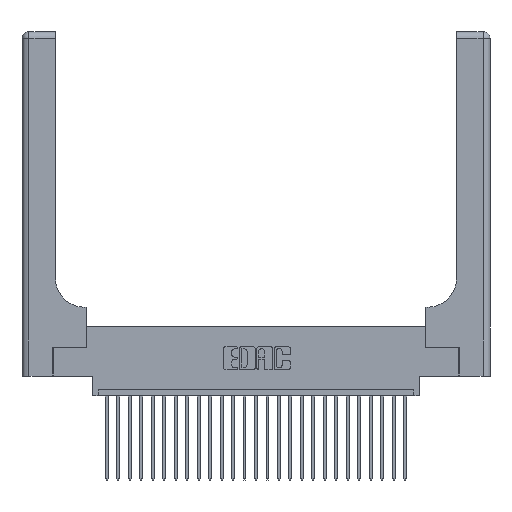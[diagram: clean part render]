
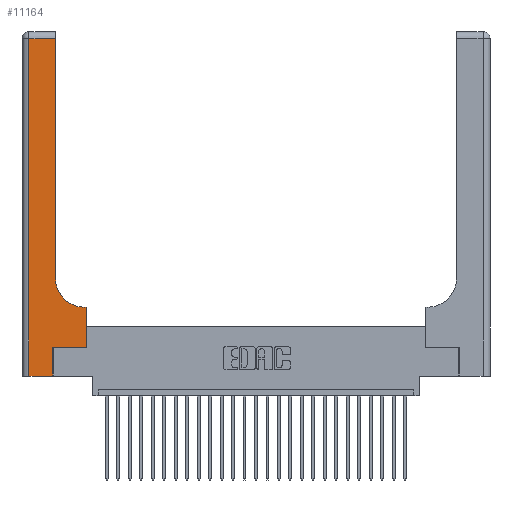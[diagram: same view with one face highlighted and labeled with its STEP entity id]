
A CAD part, top view. The second image highlights one B-rep face of the part: STEP entity #11164.
In plain terms, the highlighted planar face has unit normal (0, 0, 1).
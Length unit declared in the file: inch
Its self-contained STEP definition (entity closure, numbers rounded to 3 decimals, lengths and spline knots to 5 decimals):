
#242 = ORIENTED_EDGE ( 'NONE', *, *, #26718, .T. ) ;
#314 = ORIENTED_EDGE ( 'NONE', *, *, #1433, .T. ) ;
#430 = FACE_OUTER_BOUND ( 'NONE', #13887, .T. ) ;
#598 = EDGE_CURVE ( 'NONE', #5281, #12562, #3356, .T. ) ;
#743 = CIRCLE ( 'NONE', #6125, 0.25 ) ;
#753 = CARTESIAN_POINT ( 'NONE',  ( 0.269, 0., 0.37 ) ) ;
#837 = DIRECTION ( 'NONE',  ( 0., 1., 0. ) ) ;
#1378 = DIRECTION ( 'NONE',  ( -1., 0., 0. ) ) ;
#1433 = EDGE_CURVE ( 'NONE', #15170, #6811, #19307, .T. ) ;
#3356 = LINE ( 'NONE', #22307, #25437 ) ;
#3408 = LINE ( 'NONE', #11684, #14414 ) ;
#4269 = EDGE_CURVE ( 'NONE', #12562, #13322, #24216, .T. ) ;
#4612 = CARTESIAN_POINT ( 'NONE',  ( 0.269, 0.25, 0.37 ) ) ;
#4697 = AXIS2_PLACEMENT_3D ( 'NONE', #5460, #16264, #18452 ) ;
#4701 = ORIENTED_EDGE ( 'NONE', *, *, #17840, .T. ) ;
#5043 = ORIENTED_EDGE ( 'NONE', *, *, #20445, .T. ) ;
#5281 = VERTEX_POINT ( 'NONE', #20880 ) ;
#5336 = CARTESIAN_POINT ( 'NONE',  ( 0.2915, 0.85, 0.37 ) ) ;
#5461 = VERTEX_POINT ( 'NONE', #25775 ) ;
#5460 = CARTESIAN_POINT ( 'NONE',  ( 0., 3., 0.37 ) ) ;
#5599 = CARTESIAN_POINT ( 'NONE',  ( 0., 0., 0.37 ) ) ;
#6125 = AXIS2_PLACEMENT_3D ( 'NONE', #19840, #26331, #11038 ) ;
#6410 = LINE ( 'NONE', #22202, #8734 ) ;
#6789 = VECTOR ( 'NONE', #22715, 39.37008 ) ;
#6811 = VERTEX_POINT ( 'NONE', #27147 ) ;
#8466 = ORIENTED_EDGE ( 'NONE', *, *, #4269, .T. ) ;
#8581 = CARTESIAN_POINT ( 'NONE',  ( 0.06, 0., 0.37 ) ) ;
#8734 = VECTOR ( 'NONE', #837, 39.37008 ) ;
#10805 = CARTESIAN_POINT ( 'NONE',  ( 0.5585, 0.6, 0.37 ) ) ;
#11038 = DIRECTION ( 'NONE',  ( 1., 0., 0. ) ) ;
#11164 = ADVANCED_FACE ( 'NONE', ( #430 ), #22750, .F. ) ;
#11684 = CARTESIAN_POINT ( 'NONE',  ( 0., 2.94, 0.37 ) ) ;
#12562 = VERTEX_POINT ( 'NONE', #8581 ) ;
#12985 = CARTESIAN_POINT ( 'NONE',  ( 0.2915, 0.6, 0.37 ) ) ;
#13123 = VECTOR ( 'NONE', #14630, 39.37008 ) ;
#13152 = ORIENTED_EDGE ( 'NONE', *, *, #15924, .T. ) ;
#13322 = VERTEX_POINT ( 'NONE', #753 ) ;
#13780 = VECTOR ( 'NONE', #22208, 39.37008 ) ;
#13887 = EDGE_LOOP ( 'NONE', ( #14535, #24738, #14708, #8466, #242, #314, #13152, #4701, #5043 ) ) ;
#14414 = VECTOR ( 'NONE', #1378, 39.37008 ) ;
#14535 = ORIENTED_EDGE ( 'NONE', *, *, #26305, .T. ) ;
#14630 = DIRECTION ( 'NONE',  ( 0., 1., 0. ) ) ;
#14708 = ORIENTED_EDGE ( 'NONE', *, *, #598, .T. ) ;
#15170 = VERTEX_POINT ( 'NONE', #23358 ) ;
#15924 = EDGE_CURVE ( 'NONE', #6811, #21618, #6410, .T. ) ;
#16187 = DIRECTION ( 'NONE',  ( 0., -1., 0. ) ) ;
#16264 = DIRECTION ( 'NONE',  ( 0., 0., -1. ) ) ;
#16613 = VERTEX_POINT ( 'NONE', #5336 ) ;
#16877 = CARTESIAN_POINT ( 'NONE',  ( 0.2915, 3., 0.37 ) ) ;
#17840 = EDGE_CURVE ( 'NONE', #21618, #20146, #26721, .T. ) ;
#18452 = DIRECTION ( 'NONE',  ( -1., 0., 0. ) ) ;
#18837 = LINE ( 'NONE', #16877, #13123 ) ;
#19017 = CARTESIAN_POINT ( 'NONE',  ( 0.5415, 0.6, 0.37 ) ) ;
#19307 = LINE ( 'NONE', #4612, #20643 ) ;
#19432 = EDGE_CURVE ( 'NONE', #5461, #5281, #3408, .T. ) ;
#19456 = DIRECTION ( 'NONE',  ( 1., 0., 0. ) ) ;
#19467 = LINE ( 'NONE', #22116, #13780 ) ;
#19840 = CARTESIAN_POINT ( 'NONE',  ( 0.5415, 0.85, 0.37 ) ) ;
#20146 = VERTEX_POINT ( 'NONE', #19017 ) ;
#20445 = EDGE_CURVE ( 'NONE', #20146, #16613, #743, .T. ) ;
#20643 = VECTOR ( 'NONE', #19456, 39.37008 ) ;
#20880 = CARTESIAN_POINT ( 'NONE',  ( 0.06, 2.94, 0.37 ) ) ;
#21618 = VERTEX_POINT ( 'NONE', #10805 ) ;
#22116 = CARTESIAN_POINT ( 'NONE',  ( 0.269, 0., 0.37 ) ) ;
#22202 = CARTESIAN_POINT ( 'NONE',  ( 0.5585, 0.25, 0.37 ) ) ;
#22208 = DIRECTION ( 'NONE',  ( 0., 1., 0. ) ) ;
#22307 = CARTESIAN_POINT ( 'NONE',  ( 0.06, 3., 0.37 ) ) ;
#22715 = DIRECTION ( 'NONE',  ( 1., 0., 0. ) ) ;
#22750 = PLANE ( 'NONE',  #4697 ) ;
#23358 = CARTESIAN_POINT ( 'NONE',  ( 0.269, 0.25, 0.37 ) ) ;
#24216 = LINE ( 'NONE', #5599, #6789 ) ;
#24702 = VECTOR ( 'NONE', #25483, 39.37008 ) ;
#24738 = ORIENTED_EDGE ( 'NONE', *, *, #19432, .T. ) ;
#25437 = VECTOR ( 'NONE', #16187, 39.37008 ) ;
#25483 = DIRECTION ( 'NONE',  ( -1., 0., 0. ) ) ;
#25775 = CARTESIAN_POINT ( 'NONE',  ( 0.2915, 2.94, 0.37 ) ) ;
#26305 = EDGE_CURVE ( 'NONE', #16613, #5461, #18837, .T. ) ;
#26331 = DIRECTION ( 'NONE',  ( 0., 0., -1. ) ) ;
#26718 = EDGE_CURVE ( 'NONE', #13322, #15170, #19467, .T. ) ;
#26721 = LINE ( 'NONE', #12985, #24702 ) ;
#27147 = CARTESIAN_POINT ( 'NONE',  ( 0.5585, 0.25, 0.37 ) ) ;
